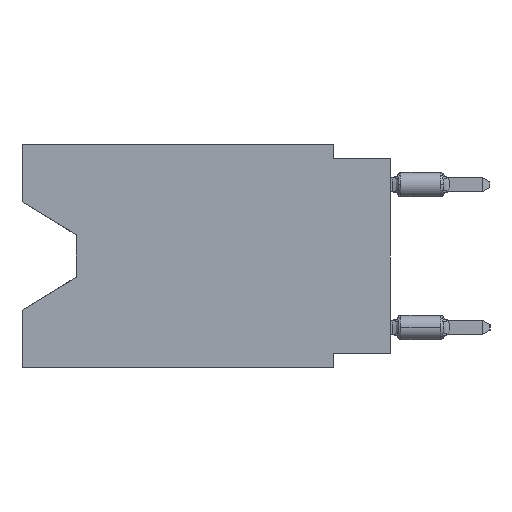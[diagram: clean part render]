
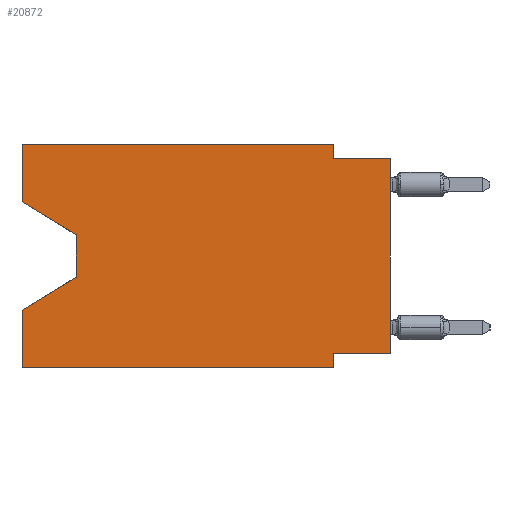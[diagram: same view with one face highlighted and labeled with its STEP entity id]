
A CAD part, left-side view. The second image highlights one B-rep face of the part: STEP entity #20872.
In plain terms, the highlighted planar face has unit normal (-1, 0, 0).
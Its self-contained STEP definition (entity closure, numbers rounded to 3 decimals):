
#542 = EDGE_CURVE ( 'NONE', #9136, #30825, #14601, .T. ) ;
#1734 = LINE ( 'NONE', #56572, #56533 ) ;
#2397 = CARTESIAN_POINT ( 'NONE',  ( 0., 2.54, -9.271 ) ) ;
#3292 = LINE ( 'NONE', #48835, #15040 ) ;
#4010 = CARTESIAN_POINT ( 'NONE',  ( 0., 2.54, 0. ) ) ;
#4159 = CARTESIAN_POINT ( 'NONE',  ( 0., 16.383, 0. ) ) ;
#4183 = DIRECTION ( 'NONE',  ( 0., 0.855, -0.519 ) ) ;
#6781 = VERTEX_POINT ( 'NONE', #33020 ) ;
#6982 = EDGE_CURVE ( 'NONE', #23557, #58277, #53354, .T. ) ;
#7342 = LINE ( 'NONE', #21157, #47980 ) ;
#7458 = EDGE_CURVE ( 'NONE', #58291, #6781, #45252, .T. ) ;
#7826 = ORIENTED_EDGE ( 'NONE', *, *, #15440, .F. ) ;
#9136 = VERTEX_POINT ( 'NONE', #54765 ) ;
#11264 = CARTESIAN_POINT ( 'NONE',  ( 0., 2.54, -0.635 ) ) ;
#11466 = CARTESIAN_POINT ( 'NONE',  ( 0., 0., 0. ) ) ;
#11505 = EDGE_CURVE ( 'NONE', #9136, #35086, #56711, .T. ) ;
#11530 = CARTESIAN_POINT ( 'NONE',  ( 0., 2.54, -9.906 ) ) ;
#12416 = LINE ( 'NONE', #4010, #26088 ) ;
#12457 = ORIENTED_EDGE ( 'NONE', *, *, #542, .F. ) ;
#14148 = EDGE_CURVE ( 'NONE', #25740, #55966, #7342, .T. ) ;
#14601 = LINE ( 'NONE', #50563, #48771 ) ;
#15040 = VECTOR ( 'NONE', #38975, 1000. ) ;
#15192 = CARTESIAN_POINT ( 'NONE',  ( 0., 16.383, -9.906 ) ) ;
#15362 = EDGE_LOOP ( 'NONE', ( #49157, #25535, #35009, #49445, #46521, #40230, #12457, #59161, #52397, #7826, #40190, #58496 ) ) ;
#15440 = EDGE_CURVE ( 'NONE', #55966, #22664, #12416, .T. ) ;
#15533 = DIRECTION ( 'NONE',  ( 0., -1., 0. ) ) ;
#17665 = DIRECTION ( 'NONE',  ( 0., 0., 1. ) ) ;
#17837 = DIRECTION ( 'NONE',  ( 0., -1., 0. ) ) ;
#18591 = VECTOR ( 'NONE', #52758, 1000. ) ;
#19106 = DIRECTION ( 'NONE',  ( 0., 1., 0. ) ) ;
#19952 = CARTESIAN_POINT ( 'NONE',  ( 0., 16.383, -2.546 ) ) ;
#20041 = CARTESIAN_POINT ( 'NONE',  ( 0., 16.383, 0. ) ) ;
#20872 = ADVANCED_FACE ( 'NONE', ( #28129 ), #32026, .F. ) ;
#21157 = CARTESIAN_POINT ( 'NONE',  ( 0., 16.383, 0. ) ) ;
#22161 = LINE ( 'NONE', #35330, #45251 ) ;
#22664 = VERTEX_POINT ( 'NONE', #11264 ) ;
#23557 = VERTEX_POINT ( 'NONE', #19952 ) ;
#23702 = EDGE_CURVE ( 'NONE', #50394, #58876, #34303, .T. ) ;
#23819 = CARTESIAN_POINT ( 'NONE',  ( 0., 13.97, -5.893 ) ) ;
#23853 = VECTOR ( 'NONE', #30998, 1000. ) ;
#25535 = ORIENTED_EDGE ( 'NONE', *, *, #45072, .T. ) ;
#25740 = VERTEX_POINT ( 'NONE', #4159 ) ;
#25912 = DIRECTION ( 'NONE',  ( 0., 0., -1. ) ) ;
#26088 = VECTOR ( 'NONE', #25912, 1000. ) ;
#27280 = CARTESIAN_POINT ( 'NONE',  ( 0., 13.97, -5.893 ) ) ;
#28129 = FACE_OUTER_BOUND ( 'NONE', #15362, .T. ) ;
#30149 = VECTOR ( 'NONE', #4183, 1000. ) ;
#30825 = VERTEX_POINT ( 'NONE', #2397 ) ;
#30849 = DIRECTION ( 'NONE',  ( 0., 0., -1. ) ) ;
#30998 = DIRECTION ( 'NONE',  ( 0., -1., 0. ) ) ;
#31965 = VECTOR ( 'NONE', #56864, 1000. ) ;
#32026 = PLANE ( 'NONE',  #37134 ) ;
#32602 = DIRECTION ( 'NONE',  ( 1., 0., 0. ) ) ;
#33020 = CARTESIAN_POINT ( 'NONE',  ( 0., 16.383, -7.36 ) ) ;
#33585 = VECTOR ( 'NONE', #52219, 1000. ) ;
#33886 = CARTESIAN_POINT ( 'NONE',  ( 0., 2.54, 0. ) ) ;
#33915 = VECTOR ( 'NONE', #30849, 1000. ) ;
#34303 = LINE ( 'NONE', #53744, #23853 ) ;
#35009 = ORIENTED_EDGE ( 'NONE', *, *, #7458, .T. ) ;
#35086 = VERTEX_POINT ( 'NONE', #49371 ) ;
#35330 = CARTESIAN_POINT ( 'NONE',  ( 0., 16.383, 0. ) ) ;
#37134 = AXIS2_PLACEMENT_3D ( 'NONE', #50293, #32602, #37393 ) ;
#37393 = DIRECTION ( 'NONE',  ( 0., 0., -1. ) ) ;
#38975 = DIRECTION ( 'NONE',  ( 0., 0., -1. ) ) ;
#40190 = ORIENTED_EDGE ( 'NONE', *, *, #14148, .F. ) ;
#40230 = ORIENTED_EDGE ( 'NONE', *, *, #48487, .F. ) ;
#41673 = EDGE_CURVE ( 'NONE', #23557, #25740, #22161, .T. ) ;
#42511 = LINE ( 'NONE', #20041, #31965 ) ;
#45072 = EDGE_CURVE ( 'NONE', #58277, #58291, #45222, .T. ) ;
#45222 = LINE ( 'NONE', #58098, #33915 ) ;
#45251 = VECTOR ( 'NONE', #17665, 1000. ) ;
#45252 = LINE ( 'NONE', #27280, #30149 ) ;
#46521 = ORIENTED_EDGE ( 'NONE', *, *, #23702, .T. ) ;
#47980 = VECTOR ( 'NONE', #17837, 1000. ) ;
#48487 = EDGE_CURVE ( 'NONE', #30825, #58876, #3292, .T. ) ;
#48771 = VECTOR ( 'NONE', #19106, 1000. ) ;
#48835 = CARTESIAN_POINT ( 'NONE',  ( 0., 2.54, -9.906 ) ) ;
#49150 = CARTESIAN_POINT ( 'NONE',  ( 0., 16.383, -2.546 ) ) ;
#49157 = ORIENTED_EDGE ( 'NONE', *, *, #6982, .T. ) ;
#49371 = CARTESIAN_POINT ( 'NONE',  ( 0., 0., -0.635 ) ) ;
#49445 = ORIENTED_EDGE ( 'NONE', *, *, #56288, .F. ) ;
#50293 = CARTESIAN_POINT ( 'NONE',  ( 0., 16.383, 0. ) ) ;
#50394 = VERTEX_POINT ( 'NONE', #15192 ) ;
#50563 = CARTESIAN_POINT ( 'NONE',  ( 0., 0., -9.271 ) ) ;
#52219 = DIRECTION ( 'NONE',  ( 0., 0., 1. ) ) ;
#52397 = ORIENTED_EDGE ( 'NONE', *, *, #52679, .F. ) ;
#52679 = EDGE_CURVE ( 'NONE', #22664, #35086, #1734, .T. ) ;
#52758 = DIRECTION ( 'NONE',  ( 0., -0.855, -0.519 ) ) ;
#53354 = LINE ( 'NONE', #49150, #18591 ) ;
#53744 = CARTESIAN_POINT ( 'NONE',  ( 0., 16.383, -9.906 ) ) ;
#54668 = CARTESIAN_POINT ( 'NONE',  ( 0., 13.97, -4.013 ) ) ;
#54765 = CARTESIAN_POINT ( 'NONE',  ( 0., 0., -9.271 ) ) ;
#55966 = VERTEX_POINT ( 'NONE', #33886 ) ;
#56288 = EDGE_CURVE ( 'NONE', #50394, #6781, #42511, .T. ) ;
#56533 = VECTOR ( 'NONE', #15533, 1000. ) ;
#56572 = CARTESIAN_POINT ( 'NONE',  ( 0., 0., -0.635 ) ) ;
#56711 = LINE ( 'NONE', #11466, #33585 ) ;
#56864 = DIRECTION ( 'NONE',  ( 0., 0., 1. ) ) ;
#58098 = CARTESIAN_POINT ( 'NONE',  ( 0., 13.97, -4.013 ) ) ;
#58277 = VERTEX_POINT ( 'NONE', #54668 ) ;
#58291 = VERTEX_POINT ( 'NONE', #23819 ) ;
#58496 = ORIENTED_EDGE ( 'NONE', *, *, #41673, .F. ) ;
#58876 = VERTEX_POINT ( 'NONE', #11530 ) ;
#59161 = ORIENTED_EDGE ( 'NONE', *, *, #11505, .T. ) ;
